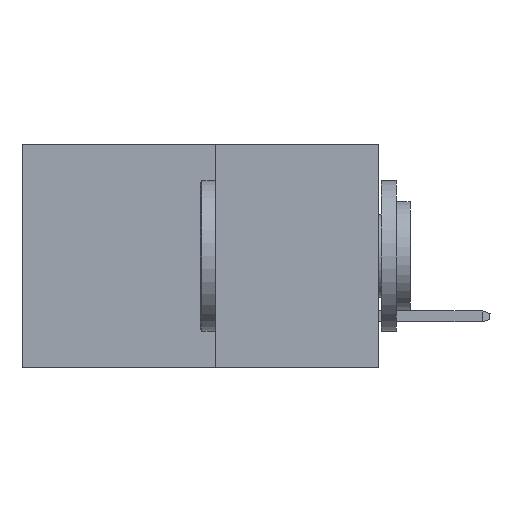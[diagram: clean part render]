
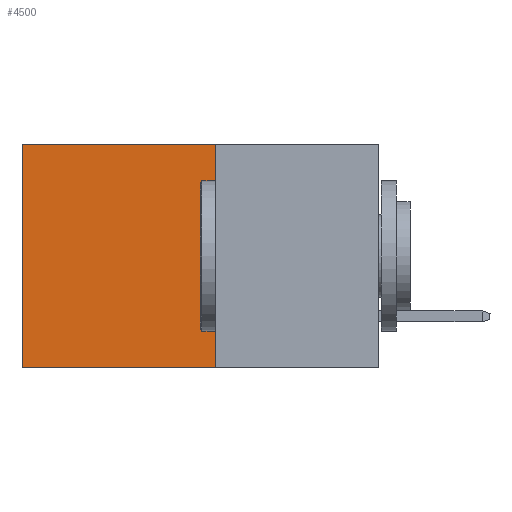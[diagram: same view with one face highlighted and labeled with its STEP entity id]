
A CAD part, left-side view. The second image highlights one B-rep face of the part: STEP entity #4500.
In plain terms, the highlighted planar face has unit normal (-1, 0, 0).
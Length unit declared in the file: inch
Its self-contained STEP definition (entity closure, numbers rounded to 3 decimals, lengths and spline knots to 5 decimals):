
#2786 = EDGE_CURVE ( 'NONE', #18946, #11646, #22439, .T. ) ;
#4500 = ADVANCED_FACE ( 'NONE', ( #22940 ), #11806, .F. ) ;
#4706 = CARTESIAN_POINT ( 'NONE',  ( 0.277, 0.27, 0. ) ) ;
#4902 = DIRECTION ( 'NONE',  ( 0., 1., 0. ) ) ;
#5605 = CARTESIAN_POINT ( 'NONE',  ( 0.277, 0.27, 0. ) ) ;
#5849 = CARTESIAN_POINT ( 'NONE',  ( 0.277, 0.59, -0.37 ) ) ;
#5887 = ORIENTED_EDGE ( 'NONE', *, *, #20569, .F. ) ;
#5976 = CARTESIAN_POINT ( 'NONE',  ( 0.277, 0.27, -0.37 ) ) ;
#6256 = VECTOR ( 'NONE', #14185, 39.37008 ) ;
#6436 = CARTESIAN_POINT ( 'NONE',  ( 0.277, 0.27, -0.37 ) ) ;
#8428 = EDGE_CURVE ( 'NONE', #11646, #14643, #21291, .T. ) ;
#10370 = VECTOR ( 'NONE', #4902, 39.37008 ) ;
#11646 = VERTEX_POINT ( 'NONE', #22831 ) ;
#11746 = DIRECTION ( 'NONE',  ( 1., 0., 0. ) ) ;
#11806 = PLANE ( 'NONE',  #19336 ) ;
#12318 = LINE ( 'NONE', #27510, #6256 ) ;
#13108 = EDGE_CURVE ( 'NONE', #18946, #17243, #12318, .T. ) ;
#13497 = DIRECTION ( 'NONE',  ( 0., 0., -1. ) ) ;
#14185 = DIRECTION ( 'NONE',  ( 0., 0., -1. ) ) ;
#14643 = VERTEX_POINT ( 'NONE', #5849 ) ;
#14847 = LINE ( 'NONE', #17583, #20159 ) ;
#14892 = CARTESIAN_POINT ( 'NONE',  ( 0.277, 0.59, -0.37 ) ) ;
#15161 = ORIENTED_EDGE ( 'NONE', *, *, #8428, .T. ) ;
#15490 = ORIENTED_EDGE ( 'NONE', *, *, #13108, .F. ) ;
#17158 = DIRECTION ( 'NONE',  ( 0., 0., -1. ) ) ;
#17243 = VERTEX_POINT ( 'NONE', #5976 ) ;
#17583 = CARTESIAN_POINT ( 'NONE',  ( 0.277, 0.27, -0.37 ) ) ;
#18946 = VERTEX_POINT ( 'NONE', #5605 ) ;
#19234 = EDGE_LOOP ( 'NONE', ( #15161, #5887, #15490, #20019 ) ) ;
#19336 = AXIS2_PLACEMENT_3D ( 'NONE', #6436, #11746, #13497 ) ;
#19844 = DIRECTION ( 'NONE',  ( 0., 1., 0. ) ) ;
#20019 = ORIENTED_EDGE ( 'NONE', *, *, #2786, .T. ) ;
#20159 = VECTOR ( 'NONE', #19844, 39.37008 ) ;
#20569 = EDGE_CURVE ( 'NONE', #17243, #14643, #14847, .T. ) ;
#20572 = VECTOR ( 'NONE', #17158, 39.37008 ) ;
#21291 = LINE ( 'NONE', #14892, #20572 ) ;
#22439 = LINE ( 'NONE', #4706, #10370 ) ;
#22831 = CARTESIAN_POINT ( 'NONE',  ( 0.277, 0.59, 0. ) ) ;
#22940 = FACE_OUTER_BOUND ( 'NONE', #19234, .T. ) ;
#27510 = CARTESIAN_POINT ( 'NONE',  ( 0.277, 0.27, -0.37 ) ) ;
